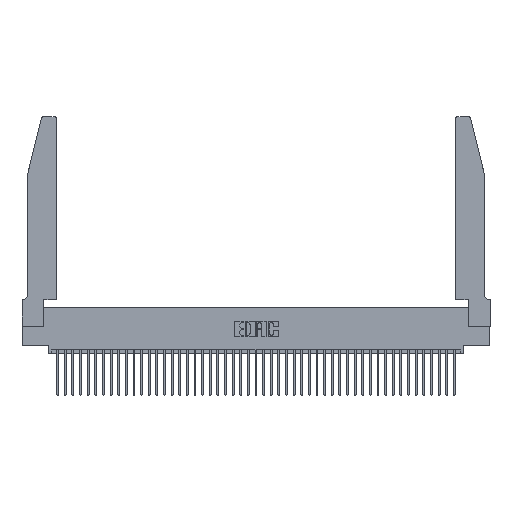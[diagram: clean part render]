
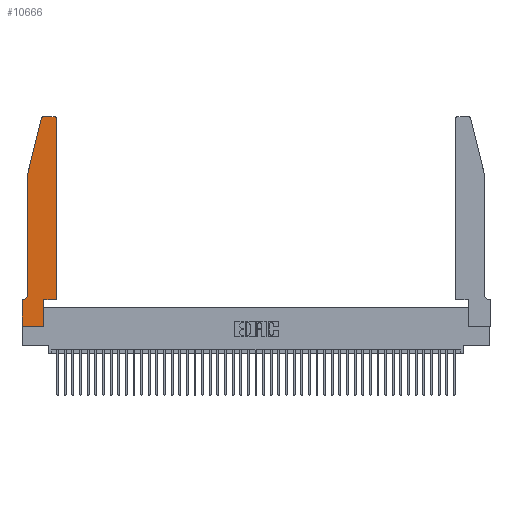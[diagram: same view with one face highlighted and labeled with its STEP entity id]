
A CAD part, top view. The second image highlights one B-rep face of the part: STEP entity #10666.
In plain terms, the highlighted planar face has unit normal (0, 0, 1).
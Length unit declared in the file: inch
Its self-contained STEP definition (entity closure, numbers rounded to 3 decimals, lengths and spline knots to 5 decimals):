
#216 = CIRCLE ( 'NONE', #43384, 0.03 ) ;
#1330 = CARTESIAN_POINT ( 'NONE',  ( 0.2865, 0.35, 0.37 ) ) ;
#1792 = CARTESIAN_POINT ( 'NONE',  ( 0.4505, 0.35, 0.37 ) ) ;
#2072 = DIRECTION ( 'NONE',  ( 1., 0., 0. ) ) ;
#2373 = VECTOR ( 'NONE', #22317, 39.37008 ) ;
#2394 = DIRECTION ( 'NONE',  ( -1., 0., 0. ) ) ;
#2490 = AXIS2_PLACEMENT_3D ( 'NONE', #40287, #29941, #2072 ) ;
#2709 = DIRECTION ( 'NONE',  ( 0., 0., 1. ) ) ;
#3099 = VERTEX_POINT ( 'NONE', #9904 ) ;
#3117 = LINE ( 'NONE', #13151, #39007 ) ;
#3242 = ORIENTED_EDGE ( 'NONE', *, *, #19975, .T. ) ;
#3247 = VERTEX_POINT ( 'NONE', #17139 ) ;
#4209 = EDGE_CURVE ( 'NONE', #9649, #19651, #10446, .T. ) ;
#4381 = CARTESIAN_POINT ( 'NONE',  ( 0.2605, 2.75, 0.37 ) ) ;
#4658 = VERTEX_POINT ( 'NONE', #16659 ) ;
#4677 = EDGE_CURVE ( 'NONE', #13240, #34813, #28840, .T. ) ;
#4971 = DIRECTION ( 'NONE',  ( 1., 0., 0. ) ) ;
#5381 = CARTESIAN_POINT ( 'NONE',  ( 0.0755, 2., 0.37 ) ) ;
#5478 = DIRECTION ( 'NONE',  ( 0., 1., 0. ) ) ;
#6019 = VECTOR ( 'NONE', #5478, 39.37008 ) ;
#6300 = CARTESIAN_POINT ( 'NONE',  ( 0., 0., 0.37 ) ) ;
#6613 = AXIS2_PLACEMENT_3D ( 'NONE', #22969, #43607, #2394 ) ;
#6745 = LINE ( 'NONE', #43430, #2373 ) ;
#7338 = CARTESIAN_POINT ( 'NONE',  ( 0.4505, 2.72, 0.37 ) ) ;
#7981 = VERTEX_POINT ( 'NONE', #43216 ) ;
#8028 = DIRECTION ( 'NONE',  ( -0.239, -0.971, 0. ) ) ;
#9028 = ORIENTED_EDGE ( 'NONE', *, *, #39137, .T. ) ;
#9649 = VERTEX_POINT ( 'NONE', #12077 ) ;
#9904 = CARTESIAN_POINT ( 'NONE',  ( 0.2865, 0., 0.37 ) ) ;
#10446 = LINE ( 'NONE', #14286, #38229 ) ;
#10666 = ADVANCED_FACE ( 'NONE', ( #18912 ), #12926, .T. ) ;
#12038 = EDGE_CURVE ( 'NONE', #34813, #3247, #216, .T. ) ;
#12077 = CARTESIAN_POINT ( 'NONE',  ( 0.25487, 2.72718, 0.37 ) ) ;
#12470 = CARTESIAN_POINT ( 'NONE',  ( 0.0755, 0.35, 0.37 ) ) ;
#12926 = PLANE ( 'NONE',  #15040 ) ;
#13151 = CARTESIAN_POINT ( 'NONE',  ( 0.4505, 0.35, 0.37 ) ) ;
#13240 = VERTEX_POINT ( 'NONE', #16385 ) ;
#13454 = DIRECTION ( 'NONE',  ( 1., 0., 0. ) ) ;
#14286 = CARTESIAN_POINT ( 'NONE',  ( 0.0755, 2., 0.37 ) ) ;
#14742 = EDGE_CURVE ( 'NONE', #3247, #28501, #23490, .T. ) ;
#15040 = AXIS2_PLACEMENT_3D ( 'NONE', #27231, #2709, #16735 ) ;
#15120 = CARTESIAN_POINT ( 'NONE',  ( 0.284, 2.75, 0.37 ) ) ;
#15869 = VECTOR ( 'NONE', #39712, 39.37008 ) ;
#16385 = CARTESIAN_POINT ( 'NONE',  ( 0.4505, 0.35, 0.37 ) ) ;
#16451 = LINE ( 'NONE', #36045, #44707 ) ;
#16659 = CARTESIAN_POINT ( 'NONE',  ( 0.0755, 0.42, 0.37 ) ) ;
#16735 = DIRECTION ( 'NONE',  ( 1., 0., 0. ) ) ;
#17139 = CARTESIAN_POINT ( 'NONE',  ( 0.4205, 2.75, 0.37 ) ) ;
#17794 = LINE ( 'NONE', #12470, #39003 ) ;
#18222 = DIRECTION ( 'NONE',  ( 0., 1., 0. ) ) ;
#18386 = VERTEX_POINT ( 'NONE', #36029 ) ;
#18734 = ORIENTED_EDGE ( 'NONE', *, *, #4677, .T. ) ;
#18895 = EDGE_CURVE ( 'NONE', #28501, #9649, #40541, .T. ) ;
#18912 = FACE_OUTER_BOUND ( 'NONE', #31479, .T. ) ;
#19651 = VERTEX_POINT ( 'NONE', #5381 ) ;
#19975 = EDGE_CURVE ( 'NONE', #19651, #4658, #16451, .T. ) ;
#20556 = ORIENTED_EDGE ( 'NONE', *, *, #4209, .T. ) ;
#22317 = DIRECTION ( 'NONE',  ( 1., 0., 0. ) ) ;
#22969 = CARTESIAN_POINT ( 'NONE',  ( 0.0055, 0.42, 0.37 ) ) ;
#23490 = LINE ( 'NONE', #4381, #15869 ) ;
#23856 = ORIENTED_EDGE ( 'NONE', *, *, #36414, .T. ) ;
#24225 = LINE ( 'NONE', #6300, #31718 ) ;
#25493 = ORIENTED_EDGE ( 'NONE', *, *, #43319, .T. ) ;
#26204 = EDGE_CURVE ( 'NONE', #18386, #40092, #24225, .T. ) ;
#26448 = CARTESIAN_POINT ( 'NONE',  ( 0.2865, 0.35, 0.37 ) ) ;
#26990 = DIRECTION ( 'NONE',  ( 0., -1., 0. ) ) ;
#27231 = CARTESIAN_POINT ( 'NONE',  ( 0., 0.35, 0.37 ) ) ;
#28501 = VERTEX_POINT ( 'NONE', #15120 ) ;
#28840 = LINE ( 'NONE', #1792, #6019 ) ;
#29276 = VECTOR ( 'NONE', #18222, 39.37008 ) ;
#29498 = DIRECTION ( 'NONE',  ( -1., 0., 0. ) ) ;
#29941 = DIRECTION ( 'NONE',  ( 0., 0., 1. ) ) ;
#30824 = ORIENTED_EDGE ( 'NONE', *, *, #33732, .T. ) ;
#31435 = LINE ( 'NONE', #1330, #29276 ) ;
#31479 = EDGE_LOOP ( 'NONE', ( #35595, #36218, #20556, #3242, #9028, #30824, #34370, #23856, #25493, #37477, #18734, #38782 ) ) ;
#31718 = VECTOR ( 'NONE', #37346, 39.37008 ) ;
#33732 = EDGE_CURVE ( 'NONE', #7981, #18386, #17794, .T. ) ;
#34342 = VERTEX_POINT ( 'NONE', #26448 ) ;
#34370 = ORIENTED_EDGE ( 'NONE', *, *, #26204, .T. ) ;
#34813 = VERTEX_POINT ( 'NONE', #7338 ) ;
#35595 = ORIENTED_EDGE ( 'NONE', *, *, #14742, .T. ) ;
#35809 = CARTESIAN_POINT ( 'NONE',  ( 0.4205, 2.72, 0.37 ) ) ;
#36029 = CARTESIAN_POINT ( 'NONE',  ( 0., 0.35, 0.37 ) ) ;
#36045 = CARTESIAN_POINT ( 'NONE',  ( 0.0755, 2., 0.37 ) ) ;
#36218 = ORIENTED_EDGE ( 'NONE', *, *, #18895, .T. ) ;
#36414 = EDGE_CURVE ( 'NONE', #40092, #3099, #6745, .T. ) ;
#37346 = DIRECTION ( 'NONE',  ( 0., -1., 0. ) ) ;
#37477 = ORIENTED_EDGE ( 'NONE', *, *, #44737, .T. ) ;
#38229 = VECTOR ( 'NONE', #8028, 39.37008 ) ;
#38782 = ORIENTED_EDGE ( 'NONE', *, *, #12038, .T. ) ;
#39003 = VECTOR ( 'NONE', #29498, 39.37008 ) ;
#39007 = VECTOR ( 'NONE', #13454, 39.37008 ) ;
#39137 = EDGE_CURVE ( 'NONE', #4658, #7981, #41635, .T. ) ;
#39712 = DIRECTION ( 'NONE',  ( -1., 0., 0. ) ) ;
#40092 = VERTEX_POINT ( 'NONE', #44322 ) ;
#40287 = CARTESIAN_POINT ( 'NONE',  ( 0.284, 2.72, 0.37 ) ) ;
#40541 = CIRCLE ( 'NONE', #2490, 0.03 ) ;
#41635 = CIRCLE ( 'NONE', #6613, 0.07 ) ;
#42979 = DIRECTION ( 'NONE',  ( 0., 0., 1. ) ) ;
#43216 = CARTESIAN_POINT ( 'NONE',  ( 0.0055, 0.35, 0.37 ) ) ;
#43319 = EDGE_CURVE ( 'NONE', #3099, #34342, #31435, .T. ) ;
#43384 = AXIS2_PLACEMENT_3D ( 'NONE', #35809, #42979, #4971 ) ;
#43430 = CARTESIAN_POINT ( 'NONE',  ( 0., 0., 0.37 ) ) ;
#43607 = DIRECTION ( 'NONE',  ( 0., 0., -1. ) ) ;
#44322 = CARTESIAN_POINT ( 'NONE',  ( 0., 0., 0.37 ) ) ;
#44707 = VECTOR ( 'NONE', #26990, 39.37008 ) ;
#44737 = EDGE_CURVE ( 'NONE', #34342, #13240, #3117, .T. ) ;
